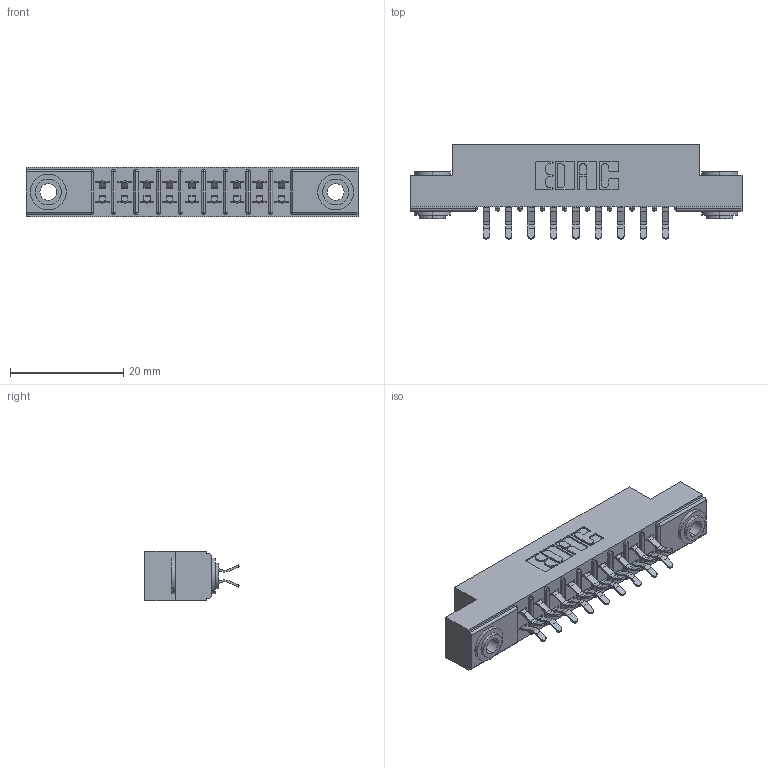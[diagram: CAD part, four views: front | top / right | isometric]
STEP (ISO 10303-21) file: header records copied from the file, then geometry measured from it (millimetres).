
FILE_DESCRIPTION (( 'STEP AP203' ), '1' );
FILE_NAME ('315-018-556-203.STEP', '2019-09-10T14:05:33', ( '' ), ( '' ), 'SwSTEP 2.0', 'SolidWorks 2016', '' );
FILE_SCHEMA (( 'CONFIG_CONTROL_DESIGN' ));
Length unit declared in the file: inch
Products named in the file (4): 315-018-556-203; 305 Part_.156 Dia; 305-290-001_556; 345-250-002_345-250-002-102
Assembly tree (21 placements, depth 2):
  315-018-556-203
    305 Part_.156 Dia
    305-290-001_556  x18
    345-250-002_345-250-002-102  x2
Bounding box: 58.67 x 16.64 x 8.71 mm (x, y, z)
Volume: 3702.2 mm3; surface area: 6469.7 mm2
Topology: 21 solids, 21 shells, 1176 faces, 3335 edges, 2170 vertices
Faces by surface type: plane 650, cylinder 482, sphere 36, cone 8
Entity records: 15049 total; most frequent: CARTESIAN_POINT 2474, ORIENTED_EDGE 2442, DIRECTION 2439, EDGE_CURVE 1221, VECTOR 937, LINE 937, VERTEX_POINT 786, AXIS2_PLACEMENT_3D 751
